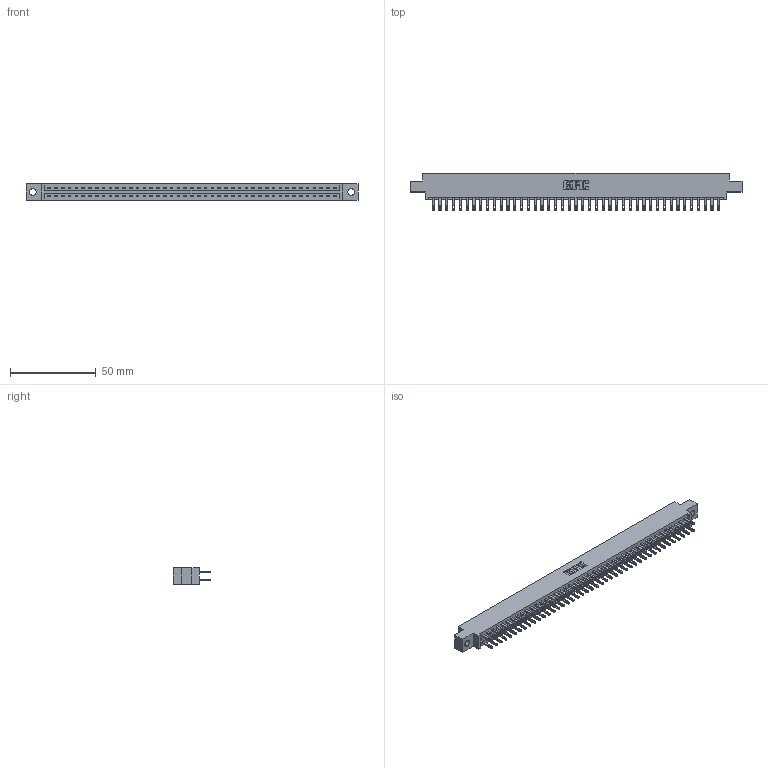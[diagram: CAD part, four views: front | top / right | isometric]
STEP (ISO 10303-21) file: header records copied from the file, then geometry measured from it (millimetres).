
FILE_DESCRIPTION (( 'STEP AP203' ), '1' );
FILE_NAME ('887-086-500-804.STEP', '2020-09-21T05:09:03', ( '' ), ( '' ), 'SwSTEP 2.0', 'SolidWorks 2020', '' );
FILE_SCHEMA (( 'CONFIG_CONTROL_DESIGN' ));
Length unit declared in the file: inch
Products named in the file (3): 345-292-001_345-293-100; 837 Part_0.170 Offset - 0.156 Dia-TH; 887-086-500-804
Assembly tree (87 placements, depth 2):
  887-086-500-804
    837 Part_0.170 Offset - 0.156 Dia-TH
    345-292-001_345-293-100  x86
Bounding box: 193.4 x 21.85 x 9.4 mm (x, y, z)
Volume: 20452.3 mm3; surface area: 23990.6 mm2
Topology: 87 solids, 87 shells, 4418 faces, 13481 edges, 8986 vertices
Faces by surface type: plane 2826, cylinder 1592
Entity records: 33275 total; most frequent: CARTESIAN_POINT 5606, ORIENTED_EDGE 5542, DIRECTION 4767, EDGE_CURVE 2771, LINE 2639, VECTOR 2639, VERTEX_POINT 1846, AXIS2_PLACEMENT_3D 1064
